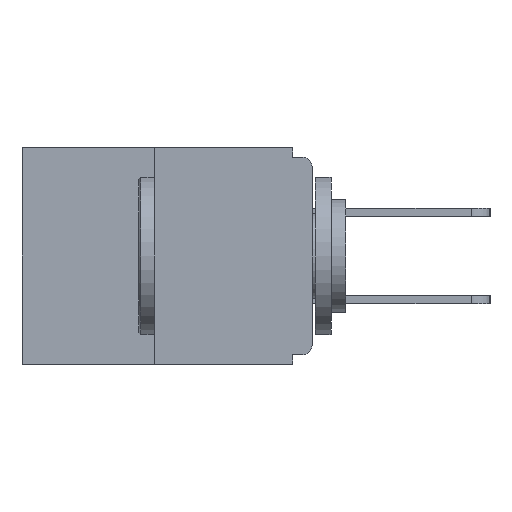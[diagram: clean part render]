
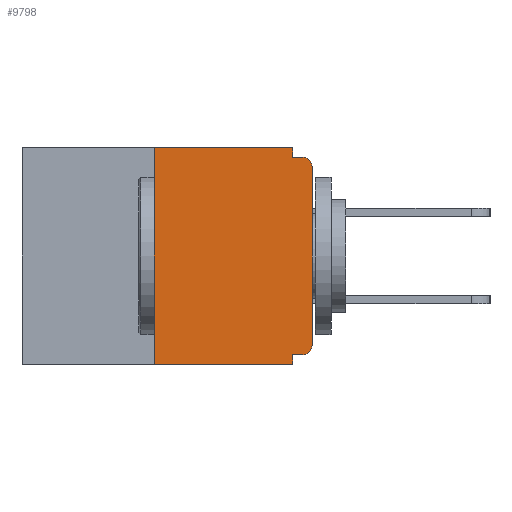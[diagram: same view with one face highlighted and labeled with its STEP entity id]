
A CAD part, left-side view. The second image highlights one B-rep face of the part: STEP entity #9798.
In plain terms, the highlighted planar face has unit normal (-1, 0, 0).
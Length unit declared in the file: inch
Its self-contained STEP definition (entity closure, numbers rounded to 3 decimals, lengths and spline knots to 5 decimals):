
#100 = DIRECTION ( 'NONE',  ( 0., 0., -1. ) ) ;
#1003 = CARTESIAN_POINT ( 'NONE',  ( 0., 0.031, -0.328 ) ) ;
#1190 = CARTESIAN_POINT ( 'NONE',  ( 0., 0.031, 0. ) ) ;
#1549 = VERTEX_POINT ( 'NONE', #1003 ) ;
#1703 = CARTESIAN_POINT ( 'NONE',  ( 0., 0.031, 0. ) ) ;
#1862 = CARTESIAN_POINT ( 'NONE',  ( 0., 0., -0.015 ) ) ;
#1897 = CARTESIAN_POINT ( 'NONE',  ( 0., 0.015, -0.03 ) ) ;
#2366 = VECTOR ( 'NONE', #9219, 39.37008 ) ;
#2433 = AXIS2_PLACEMENT_3D ( 'NONE', #21538, #8510, #12738 ) ;
#2511 = ORIENTED_EDGE ( 'NONE', *, *, #24239, .T. ) ;
#2582 = CARTESIAN_POINT ( 'NONE',  ( 0., 0.015, -0.015 ) ) ;
#5581 = VERTEX_POINT ( 'NONE', #11599 ) ;
#5901 = DIRECTION ( 'NONE',  ( 0., -1., 0. ) ) ;
#7658 = CARTESIAN_POINT ( 'NONE',  ( 0., 0.031, -0.343 ) ) ;
#7737 = CARTESIAN_POINT ( 'NONE',  ( 0., 0., 0. ) ) ;
#8072 = VERTEX_POINT ( 'NONE', #21266 ) ;
#8133 = LINE ( 'NONE', #24292, #2366 ) ;
#8178 = CARTESIAN_POINT ( 'NONE',  ( 0., 0.46, -0.343 ) ) ;
#8402 = CARTESIAN_POINT ( 'NONE',  ( 0., 0.46, 0. ) ) ;
#8510 = DIRECTION ( 'NONE',  ( 1., 0., 0. ) ) ;
#8584 = EDGE_CURVE ( 'NONE', #23126, #15922, #27300, .T. ) ;
#8796 = DIRECTION ( 'NONE',  ( -1., 0., 0. ) ) ;
#8820 = VECTOR ( 'NONE', #23643, 39.37008 ) ;
#8910 = CIRCLE ( 'NONE', #14653, 0.015 ) ;
#8915 = LINE ( 'NONE', #9306, #27091 ) ;
#9114 = ORIENTED_EDGE ( 'NONE', *, *, #13659, .F. ) ;
#9159 = DIRECTION ( 'NONE',  ( -1., 0., 0. ) ) ;
#9219 = DIRECTION ( 'NONE',  ( 0., 1., 0. ) ) ;
#9306 = CARTESIAN_POINT ( 'NONE',  ( 0., 0.031, -0.343 ) ) ;
#9317 = ORIENTED_EDGE ( 'NONE', *, *, #13564, .F. ) ;
#9798 = ADVANCED_FACE ( 'NONE', ( #16258 ), #25853, .F. ) ;
#10391 = CARTESIAN_POINT ( 'NONE',  ( 0., 0.25, 0. ) ) ;
#10563 = EDGE_LOOP ( 'NONE', ( #9317, #22171, #2511, #10790, #9114, #11229, #14849, #20418, #22352, #21770 ) ) ;
#10790 = ORIENTED_EDGE ( 'NONE', *, *, #17078, .F. ) ;
#10831 = EDGE_CURVE ( 'NONE', #22169, #23126, #18573, .T. ) ;
#11229 = ORIENTED_EDGE ( 'NONE', *, *, #17243, .T. ) ;
#11263 = VERTEX_POINT ( 'NONE', #7658 ) ;
#11526 = DIRECTION ( 'NONE',  ( 0., 0., -1. ) ) ;
#11599 = CARTESIAN_POINT ( 'NONE',  ( 0., 0.015, -0.328 ) ) ;
#12240 = CARTESIAN_POINT ( 'NONE',  ( 0., 0., -0.313 ) ) ;
#12596 = VERTEX_POINT ( 'NONE', #12240 ) ;
#12738 = DIRECTION ( 'NONE',  ( 0., 0., -1. ) ) ;
#13518 = DIRECTION ( 'NONE',  ( 0., 0., 1. ) ) ;
#13564 = EDGE_CURVE ( 'NONE', #21444, #22169, #23939, .T. ) ;
#13659 = EDGE_CURVE ( 'NONE', #5581, #1549, #8133, .T. ) ;
#13971 = DIRECTION ( 'NONE',  ( 0., 0., 1. ) ) ;
#14181 = EDGE_CURVE ( 'NONE', #21482, #21444, #16006, .T. ) ;
#14653 = AXIS2_PLACEMENT_3D ( 'NONE', #1897, #8796, #100 ) ;
#14849 = ORIENTED_EDGE ( 'NONE', *, *, #21188, .T. ) ;
#14894 = VECTOR ( 'NONE', #5901, 39.37008 ) ;
#15573 = LINE ( 'NONE', #8178, #14894 ) ;
#15652 = VECTOR ( 'NONE', #23834, 39.37008 ) ;
#15705 = DIRECTION ( 'NONE',  ( 0., 0., -1. ) ) ;
#15922 = VERTEX_POINT ( 'NONE', #2582 ) ;
#16006 = LINE ( 'NONE', #16108, #17401 ) ;
#16108 = CARTESIAN_POINT ( 'NONE',  ( 0., 0.25, 0. ) ) ;
#16258 = FACE_OUTER_BOUND ( 'NONE', #10563, .T. ) ;
#16547 = VECTOR ( 'NONE', #25789, 39.37008 ) ;
#17078 = EDGE_CURVE ( 'NONE', #1549, #11263, #8915, .T. ) ;
#17243 = EDGE_CURVE ( 'NONE', #5581, #12596, #19861, .T. ) ;
#17401 = VECTOR ( 'NONE', #13518, 39.37008 ) ;
#18094 = EDGE_CURVE ( 'NONE', #8072, #15922, #8910, .T. ) ;
#18573 = LINE ( 'NONE', #1703, #16547 ) ;
#19861 = CIRCLE ( 'NONE', #25058, 0.015 ) ;
#20418 = ORIENTED_EDGE ( 'NONE', *, *, #18094, .T. ) ;
#21188 = EDGE_CURVE ( 'NONE', #12596, #8072, #23871, .T. ) ;
#21266 = CARTESIAN_POINT ( 'NONE',  ( 0., 0., -0.03 ) ) ;
#21444 = VERTEX_POINT ( 'NONE', #10391 ) ;
#21482 = VERTEX_POINT ( 'NONE', #21696 ) ;
#21538 = CARTESIAN_POINT ( 'NONE',  ( 0., 0.46, 0. ) ) ;
#21696 = CARTESIAN_POINT ( 'NONE',  ( 0., 0.25, -0.343 ) ) ;
#21770 = ORIENTED_EDGE ( 'NONE', *, *, #10831, .F. ) ;
#22169 = VERTEX_POINT ( 'NONE', #1190 ) ;
#22171 = ORIENTED_EDGE ( 'NONE', *, *, #14181, .F. ) ;
#22352 = ORIENTED_EDGE ( 'NONE', *, *, #8584, .F. ) ;
#23126 = VERTEX_POINT ( 'NONE', #23874 ) ;
#23643 = DIRECTION ( 'NONE',  ( 0., -1., 0. ) ) ;
#23834 = DIRECTION ( 'NONE',  ( 0., -1., 0. ) ) ;
#23871 = LINE ( 'NONE', #7737, #27302 ) ;
#23874 = CARTESIAN_POINT ( 'NONE',  ( 0., 0.031, -0.015 ) ) ;
#23939 = LINE ( 'NONE', #8402, #8820 ) ;
#24239 = EDGE_CURVE ( 'NONE', #21482, #11263, #15573, .T. ) ;
#24292 = CARTESIAN_POINT ( 'NONE',  ( 0., 0., -0.328 ) ) ;
#25058 = AXIS2_PLACEMENT_3D ( 'NONE', #26981, #9159, #15705 ) ;
#25789 = DIRECTION ( 'NONE',  ( 0., 0., -1. ) ) ;
#25853 = PLANE ( 'NONE',  #2433 ) ;
#26981 = CARTESIAN_POINT ( 'NONE',  ( 0., 0.015, -0.313 ) ) ;
#27091 = VECTOR ( 'NONE', #11526, 39.37008 ) ;
#27300 = LINE ( 'NONE', #1862, #15652 ) ;
#27302 = VECTOR ( 'NONE', #13971, 39.37008 ) ;
